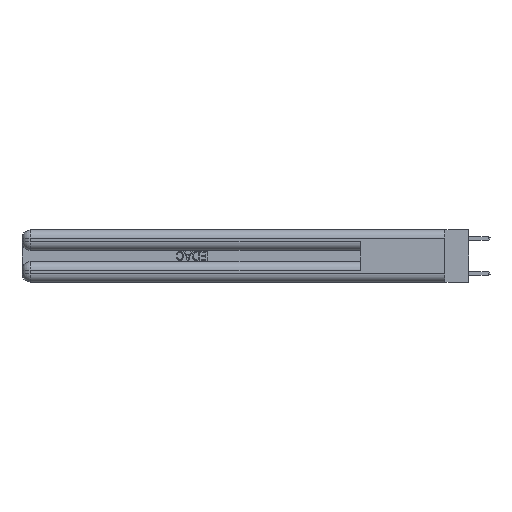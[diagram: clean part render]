
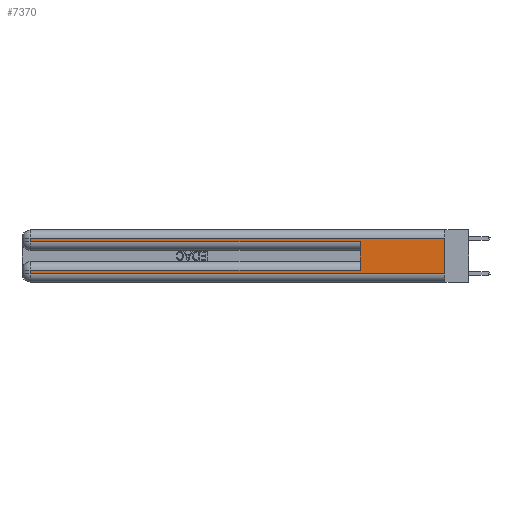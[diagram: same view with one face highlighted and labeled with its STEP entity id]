
A CAD part, left-side view. The second image highlights one B-rep face of the part: STEP entity #7370.
In plain terms, the highlighted planar face has unit normal (-1, 0, 0).
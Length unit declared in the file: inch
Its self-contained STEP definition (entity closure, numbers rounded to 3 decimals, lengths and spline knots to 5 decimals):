
#99 = FACE_OUTER_BOUND ( 'NONE', #11106, .T. ) ;
#596 = DIRECTION ( 'NONE',  ( 0., 0., -1. ) ) ;
#731 = LINE ( 'NONE', #1042, #11983 ) ;
#1012 = ORIENTED_EDGE ( 'NONE', *, *, #2297, .T. ) ;
#1042 = CARTESIAN_POINT ( 'NONE',  ( 0., 0., 0.31 ) ) ;
#1052 = VERTEX_POINT ( 'NONE', #14925 ) ;
#1171 = CARTESIAN_POINT ( 'NONE',  ( 0., 2.94, 0.285 ) ) ;
#1673 = CARTESIAN_POINT ( 'NONE',  ( 0., 0.6, 0.085 ) ) ;
#2297 = EDGE_CURVE ( 'NONE', #7997, #1052, #21584, .T. ) ;
#2370 = DIRECTION ( 'NONE',  ( 0., -1., 0. ) ) ;
#2484 = EDGE_CURVE ( 'NONE', #28979, #4740, #731, .T. ) ;
#2747 = DIRECTION ( 'NONE',  ( 0., 0., -1. ) ) ;
#3081 = DIRECTION ( 'NONE',  ( 0., 1., 0. ) ) ;
#3318 = CARTESIAN_POINT ( 'NONE',  ( 0., 0., 0.37 ) ) ;
#3356 = ORIENTED_EDGE ( 'NONE', *, *, #21976, .T. ) ;
#3822 = VERTEX_POINT ( 'NONE', #1673 ) ;
#4248 = CARTESIAN_POINT ( 'NONE',  ( 0., 2.94, 0.06 ) ) ;
#4740 = VERTEX_POINT ( 'NONE', #14421 ) ;
#6884 = VECTOR ( 'NONE', #596, 39.37008 ) ;
#7370 = ADVANCED_FACE ( 'NONE', ( #99 ), #9865, .F. ) ;
#7397 = VECTOR ( 'NONE', #13043, 39.37008 ) ;
#7453 = CARTESIAN_POINT ( 'NONE',  ( 0., 2.94, 0.37 ) ) ;
#7997 = VERTEX_POINT ( 'NONE', #4248 ) ;
#8026 = VERTEX_POINT ( 'NONE', #28104 ) ;
#8381 = ORIENTED_EDGE ( 'NONE', *, *, #2484, .T. ) ;
#9503 = DIRECTION ( 'NONE',  ( 0., 0., -1. ) ) ;
#9773 = CARTESIAN_POINT ( 'NONE',  ( 0., 0., 0.285 ) ) ;
#9865 = PLANE ( 'NONE',  #17859 ) ;
#11106 = EDGE_LOOP ( 'NONE', ( #19904, #8381, #18320, #11117, #22971, #3356, #12194, #1012 ) ) ;
#11117 = ORIENTED_EDGE ( 'NONE', *, *, #31026, .T. ) ;
#11832 = VECTOR ( 'NONE', #9503, 39.37008 ) ;
#11983 = VECTOR ( 'NONE', #3081, 39.37008 ) ;
#12144 = CARTESIAN_POINT ( 'NONE',  ( 0., 2.94, 0.37 ) ) ;
#12194 = ORIENTED_EDGE ( 'NONE', *, *, #24418, .T. ) ;
#12347 = LINE ( 'NONE', #7453, #11832 ) ;
#12457 = VECTOR ( 'NONE', #17004, 39.37008 ) ;
#12549 = CARTESIAN_POINT ( 'NONE',  ( 0., 0., 0.31 ) ) ;
#13043 = DIRECTION ( 'NONE',  ( 0., 1., 0. ) ) ;
#14421 = CARTESIAN_POINT ( 'NONE',  ( 0., 2.94, 0.31 ) ) ;
#14925 = CARTESIAN_POINT ( 'NONE',  ( 0., 0., 0.06 ) ) ;
#15676 = DIRECTION ( 'NONE',  ( 0., 0., 1. ) ) ;
#17004 = DIRECTION ( 'NONE',  ( 0., -1., 0. ) ) ;
#17023 = LINE ( 'NONE', #12144, #6884 ) ;
#17129 = DIRECTION ( 'NONE',  ( 1., 0., 0. ) ) ;
#17699 = LINE ( 'NONE', #3318, #17845 ) ;
#17845 = VECTOR ( 'NONE', #17847, 39.37008 ) ;
#17847 = DIRECTION ( 'NONE',  ( 0., 0., -1. ) ) ;
#17859 = AXIS2_PLACEMENT_3D ( 'NONE', #19028, #17129, #2747 ) ;
#17906 = CARTESIAN_POINT ( 'NONE',  ( 0., 0., 0.085 ) ) ;
#18194 = LINE ( 'NONE', #20418, #27345 ) ;
#18320 = ORIENTED_EDGE ( 'NONE', *, *, #27049, .T. ) ;
#18454 = CARTESIAN_POINT ( 'NONE',  ( 0., 0.6, 0.285 ) ) ;
#19028 = CARTESIAN_POINT ( 'NONE',  ( 0., 0., 0.37 ) ) ;
#19904 = ORIENTED_EDGE ( 'NONE', *, *, #30735, .F. ) ;
#20418 = CARTESIAN_POINT ( 'NONE',  ( 0., 0.6, 0.145 ) ) ;
#21584 = LINE ( 'NONE', #21889, #12457 ) ;
#21889 = CARTESIAN_POINT ( 'NONE',  ( 0., 0., 0.06 ) ) ;
#21976 = EDGE_CURVE ( 'NONE', #3822, #8026, #27365, .T. ) ;
#22971 = ORIENTED_EDGE ( 'NONE', *, *, #29098, .F. ) ;
#23917 = VECTOR ( 'NONE', #2370, 39.37008 ) ;
#24257 = VERTEX_POINT ( 'NONE', #18454 ) ;
#24418 = EDGE_CURVE ( 'NONE', #8026, #7997, #17023, .T. ) ;
#25175 = VERTEX_POINT ( 'NONE', #1171 ) ;
#26192 = LINE ( 'NONE', #9773, #23917 ) ;
#27049 = EDGE_CURVE ( 'NONE', #4740, #25175, #12347, .T. ) ;
#27345 = VECTOR ( 'NONE', #15676, 39.37008 ) ;
#27365 = LINE ( 'NONE', #17906, #7397 ) ;
#28104 = CARTESIAN_POINT ( 'NONE',  ( 0., 2.94, 0.085 ) ) ;
#28979 = VERTEX_POINT ( 'NONE', #12549 ) ;
#29098 = EDGE_CURVE ( 'NONE', #3822, #24257, #18194, .T. ) ;
#30735 = EDGE_CURVE ( 'NONE', #28979, #1052, #17699, .T. ) ;
#31026 = EDGE_CURVE ( 'NONE', #25175, #24257, #26192, .T. ) ;
